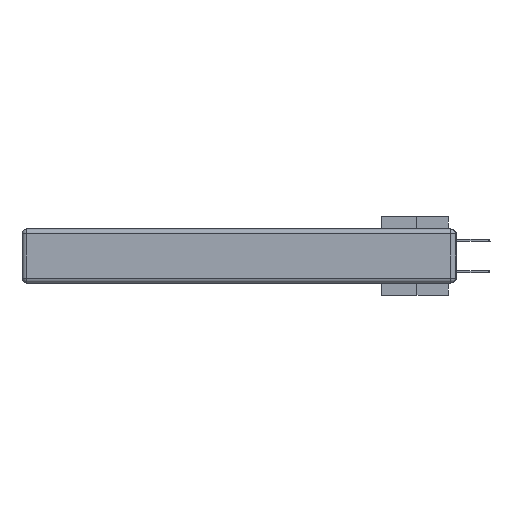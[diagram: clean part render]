
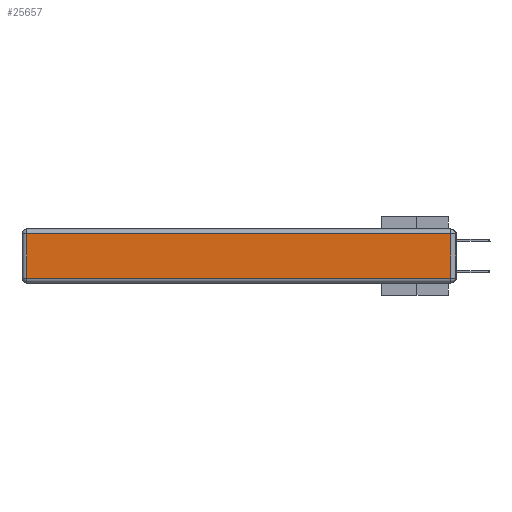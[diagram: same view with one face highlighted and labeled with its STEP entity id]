
A CAD part, left-side view. The second image highlights one B-rep face of the part: STEP entity #25657.
In plain terms, the highlighted planar face has unit normal (-1, 0, 0).
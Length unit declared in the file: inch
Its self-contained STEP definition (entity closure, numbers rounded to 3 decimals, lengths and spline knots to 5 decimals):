
#215 = VERTEX_POINT ( 'NONE', #23703 ) ;
#794 = CARTESIAN_POINT ( 'NONE',  ( 0., 2.75, -0.03 ) ) ;
#994 = LINE ( 'NONE', #794, #22347 ) ;
#1191 = VECTOR ( 'NONE', #36763, 39.37008 ) ;
#1249 = VECTOR ( 'NONE', #35793, 39.37008 ) ;
#1424 = ORIENTED_EDGE ( 'NONE', *, *, #25808, .T. ) ;
#3182 = AXIS2_PLACEMENT_3D ( 'NONE', #39974, #37144, #12147 ) ;
#5423 = VERTEX_POINT ( 'NONE', #32600 ) ;
#6061 = FACE_OUTER_BOUND ( 'NONE', #23066, .T. ) ;
#6540 = VERTEX_POINT ( 'NONE', #13133 ) ;
#7762 = CARTESIAN_POINT ( 'NONE',  ( 0., 0.03, -0.343 ) ) ;
#9890 = LINE ( 'NONE', #32006, #27819 ) ;
#12147 = DIRECTION ( 'NONE',  ( 0., 0., 1. ) ) ;
#13133 = CARTESIAN_POINT ( 'NONE',  ( 0., 0.03, -0.03 ) ) ;
#13641 = ORIENTED_EDGE ( 'NONE', *, *, #26920, .T. ) ;
#15038 = CARTESIAN_POINT ( 'NONE',  ( 0., 2.72, -0.03 ) ) ;
#16387 = ORIENTED_EDGE ( 'NONE', *, *, #27887, .T. ) ;
#21582 = EDGE_CURVE ( 'NONE', #6540, #23815, #994, .T. ) ;
#21689 = LINE ( 'NONE', #24369, #1191 ) ;
#22271 = DIRECTION ( 'NONE',  ( 0., -1., 0. ) ) ;
#22347 = VECTOR ( 'NONE', #35296, 39.37008 ) ;
#22992 = LINE ( 'NONE', #7762, #1249 ) ;
#23066 = EDGE_LOOP ( 'NONE', ( #1424, #16387, #28761, #13641 ) ) ;
#23703 = CARTESIAN_POINT ( 'NONE',  ( 0., 2.72, -0.313 ) ) ;
#23815 = VERTEX_POINT ( 'NONE', #15038 ) ;
#24369 = CARTESIAN_POINT ( 'NONE',  ( 0., 2.72, -0.343 ) ) ;
#25657 = ADVANCED_FACE ( 'NONE', ( #6061 ), #30826, .T. ) ;
#25808 = EDGE_CURVE ( 'NONE', #215, #5423, #9890, .T. ) ;
#26920 = EDGE_CURVE ( 'NONE', #23815, #215, #21689, .T. ) ;
#27819 = VECTOR ( 'NONE', #22271, 39.37008 ) ;
#27887 = EDGE_CURVE ( 'NONE', #5423, #6540, #22992, .T. ) ;
#28761 = ORIENTED_EDGE ( 'NONE', *, *, #21582, .T. ) ;
#30826 = PLANE ( 'NONE',  #3182 ) ;
#32006 = CARTESIAN_POINT ( 'NONE',  ( 0., 0., -0.313 ) ) ;
#32600 = CARTESIAN_POINT ( 'NONE',  ( 0., 0.03, -0.313 ) ) ;
#35296 = DIRECTION ( 'NONE',  ( 0., 1., 0. ) ) ;
#35793 = DIRECTION ( 'NONE',  ( 0., 0., 1. ) ) ;
#36763 = DIRECTION ( 'NONE',  ( 0., 0., -1. ) ) ;
#37144 = DIRECTION ( 'NONE',  ( -1., 0., 0. ) ) ;
#39974 = CARTESIAN_POINT ( 'NONE',  ( 0., 0., -0.343 ) ) ;
